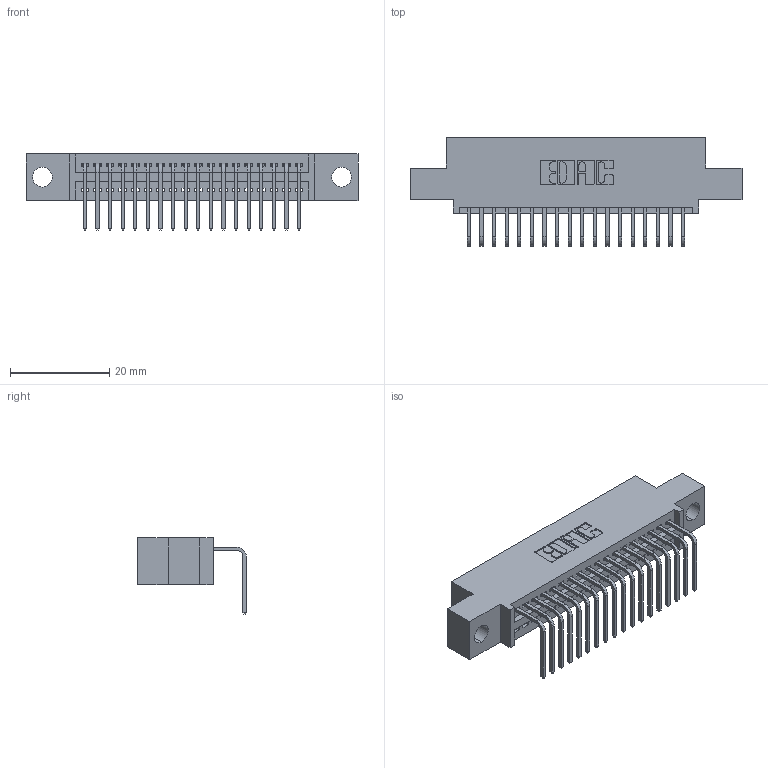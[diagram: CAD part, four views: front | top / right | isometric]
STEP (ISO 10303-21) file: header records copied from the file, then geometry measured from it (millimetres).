
FILE_DESCRIPTION (( 'STEP AP203' ), '1' );
FILE_NAME ('395-018-558-404.STEP', '2021-06-11T14:11:37', ( '' ), ( '' ), 'SwSTEP 2.0', 'SolidWorks 2020', '' );
FILE_SCHEMA (( 'CONFIG_CONTROL_DESIGN' ));
Length unit declared in the file: inch
Products named in the file (3): 345 Part_0.110 Offset - 0.156 Dia-TI; 345-292-001_558 Tail - 2; 395-018-558-404
Assembly tree (19 placements, depth 2):
  395-018-558-404
    345 Part_0.110 Offset - 0.156 Dia-TI
    345-292-001_558 Tail - 2  x18
Bounding box: 66.93 x 21.83 x 15.37 mm (x, y, z)
Volume: 6041 mm3; surface area: 7978.6 mm2
Topology: 19 solids, 19 shells, 1224 faces, 3665 edges, 2418 vertices
Faces by surface type: plane 854, cylinder 370
Entity records: 17413 total; most frequent: CARTESIAN_POINT 3028, ORIENTED_EDGE 2978, DIRECTION 2677, EDGE_CURVE 1489, VECTOR 1285, LINE 1285, VERTEX_POINT 990, AXIS2_PLACEMENT_3D 696
